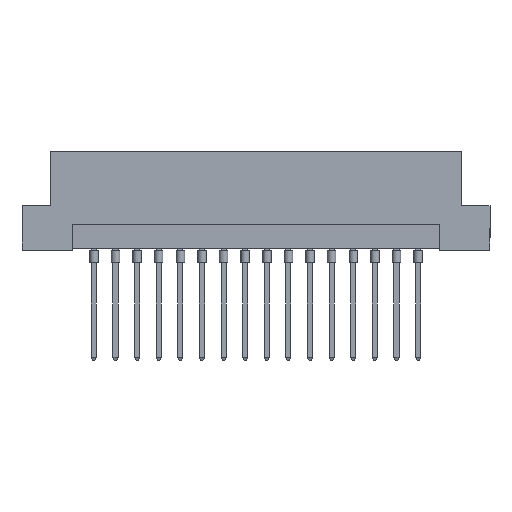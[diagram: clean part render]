
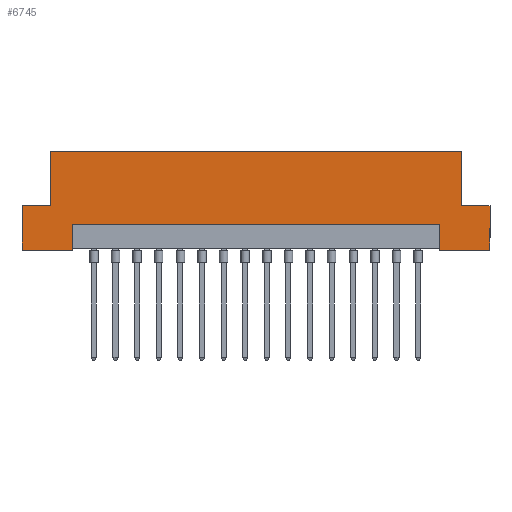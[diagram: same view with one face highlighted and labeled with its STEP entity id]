
A CAD part, front view. The second image highlights one B-rep face of the part: STEP entity #6745.
In plain terms, the highlighted planar face has unit normal (0, -1, 0).
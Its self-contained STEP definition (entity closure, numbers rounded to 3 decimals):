
#138 = VERTEX_POINT ( 'NONE', #5487 ) ;
#185 = CARTESIAN_POINT ( 'NONE',  ( -27.5, -4.3, 0. ) ) ;
#204 = VERTEX_POINT ( 'NONE', #851 ) ;
#213 = EDGE_CURVE ( 'NONE', #204, #7068, #4487, .T. ) ;
#248 = EDGE_CURVE ( 'NONE', #3055, #945, #3941, .T. ) ;
#302 = LINE ( 'NONE', #2579, #6960 ) ;
#372 = EDGE_CURVE ( 'NONE', #3192, #7068, #4767, .T. ) ;
#400 = DIRECTION ( 'NONE',  ( -1., 0., 0. ) ) ;
#407 = VECTOR ( 'NONE', #2073, 1000. ) ;
#435 = DIRECTION ( 'NONE',  ( 1., 0., 0. ) ) ;
#464 = EDGE_CURVE ( 'NONE', #3206, #4541, #3808, .T. ) ;
#480 = ORIENTED_EDGE ( 'NONE', *, *, #2262, .F. ) ;
#520 = CARTESIAN_POINT ( 'NONE',  ( -24.2, -4.3, 5.2 ) ) ;
#597 = ORIENTED_EDGE ( 'NONE', *, *, #213, .F. ) ;
#606 = DIRECTION ( 'NONE',  ( 1., 0., 0. ) ) ;
#626 = DIRECTION ( 'NONE',  ( 0., 0., -1. ) ) ;
#647 = ORIENTED_EDGE ( 'NONE', *, *, #3857, .F. ) ;
#851 = CARTESIAN_POINT ( 'NONE',  ( 21.6, -4.3, 0. ) ) ;
#887 = ORIENTED_EDGE ( 'NONE', *, *, #248, .T. ) ;
#945 = VERTEX_POINT ( 'NONE', #6007 ) ;
#1149 = CARTESIAN_POINT ( 'NONE',  ( -27.5, -4.3, 11.6 ) ) ;
#1151 = DIRECTION ( 'NONE',  ( 0., 0., 1. ) ) ;
#1225 = ORIENTED_EDGE ( 'NONE', *, *, #4520, .F. ) ;
#1260 = VECTOR ( 'NONE', #606, 1000. ) ;
#1372 = LINE ( 'NONE', #6908, #6774 ) ;
#1403 = EDGE_CURVE ( 'NONE', #3192, #945, #3871, .T. ) ;
#1470 = DIRECTION ( 'NONE',  ( 0., 0., 1. ) ) ;
#1485 = ORIENTED_EDGE ( 'NONE', *, *, #372, .T. ) ;
#1517 = DIRECTION ( 'NONE',  ( 1., 0., 0. ) ) ;
#1520 = ORIENTED_EDGE ( 'NONE', *, *, #1403, .F. ) ;
#1553 = CARTESIAN_POINT ( 'NONE',  ( 27.5, -4.3, 0. ) ) ;
#1644 = CARTESIAN_POINT ( 'NONE',  ( 24.2, -4.3, 5.2 ) ) ;
#1664 = ORIENTED_EDGE ( 'NONE', *, *, #6808, .T. ) ;
#1758 = EDGE_CURVE ( 'NONE', #4231, #3804, #3648, .T. ) ;
#1940 = FACE_OUTER_BOUND ( 'NONE', #5467, .T. ) ;
#1981 = VECTOR ( 'NONE', #5628, 1000. ) ;
#2043 = CARTESIAN_POINT ( 'NONE',  ( -21.6, -4.3, 3. ) ) ;
#2073 = DIRECTION ( 'NONE',  ( 1., 0., 0. ) ) ;
#2262 = EDGE_CURVE ( 'NONE', #4231, #3206, #302, .T. ) ;
#2272 = DIRECTION ( 'NONE',  ( 0., 0., -1. ) ) ;
#2413 = VERTEX_POINT ( 'NONE', #520 ) ;
#2546 = VECTOR ( 'NONE', #1470, 1000. ) ;
#2549 = DIRECTION ( 'NONE',  ( 1., 0., 0. ) ) ;
#2579 = CARTESIAN_POINT ( 'NONE',  ( 27.5, -4.3, 5.2 ) ) ;
#2624 = VECTOR ( 'NONE', #435, 1000. ) ;
#2743 = LINE ( 'NONE', #6588, #1981 ) ;
#2784 = VECTOR ( 'NONE', #1517, 1000. ) ;
#3055 = VERTEX_POINT ( 'NONE', #185 ) ;
#3159 = CARTESIAN_POINT ( 'NONE',  ( 24.2, -4.3, 5.2 ) ) ;
#3179 = CARTESIAN_POINT ( 'NONE',  ( -21.6, -4.3, 3. ) ) ;
#3192 = VERTEX_POINT ( 'NONE', #3179 ) ;
#3206 = VERTEX_POINT ( 'NONE', #7001 ) ;
#3353 = CARTESIAN_POINT ( 'NONE',  ( 27.5, -4.3, 0. ) ) ;
#3574 = DIRECTION ( 'NONE',  ( 0., 0., 1. ) ) ;
#3604 = DIRECTION ( 'NONE',  ( 0., 1., 0. ) ) ;
#3634 = LINE ( 'NONE', #7040, #407 ) ;
#3648 = LINE ( 'NONE', #3159, #2546 ) ;
#3804 = VERTEX_POINT ( 'NONE', #7167 ) ;
#3808 = LINE ( 'NONE', #6565, #7158 ) ;
#3857 = EDGE_CURVE ( 'NONE', #5501, #2413, #2743, .T. ) ;
#3871 = LINE ( 'NONE', #5454, #5777 ) ;
#3941 = LINE ( 'NONE', #3353, #1260 ) ;
#4032 = CARTESIAN_POINT ( 'NONE',  ( 21.6, -4.3, 3. ) ) ;
#4230 = AXIS2_PLACEMENT_3D ( 'NONE', #6348, #3604, #400 ) ;
#4231 = VERTEX_POINT ( 'NONE', #1644 ) ;
#4487 = LINE ( 'NONE', #6832, #7036 ) ;
#4520 = EDGE_CURVE ( 'NONE', #138, #3804, #7034, .T. ) ;
#4541 = VERTEX_POINT ( 'NONE', #1553 ) ;
#4767 = LINE ( 'NONE', #2043, #2624 ) ;
#5176 = DIRECTION ( 'NONE',  ( 0., 0., -1. ) ) ;
#5250 = CARTESIAN_POINT ( 'NONE',  ( -27.5, -4.3, 5.2 ) ) ;
#5270 = ORIENTED_EDGE ( 'NONE', *, *, #1758, .T. ) ;
#5454 = CARTESIAN_POINT ( 'NONE',  ( -21.6, -4.3, 0.2 ) ) ;
#5458 = ORIENTED_EDGE ( 'NONE', *, *, #5891, .F. ) ;
#5467 = EDGE_LOOP ( 'NONE', ( #1485, #597, #1664, #6492, #480, #5270, #1225, #5458, #647, #5688, #887, #1520 ) ) ;
#5487 = CARTESIAN_POINT ( 'NONE',  ( -24.2, -4.3, 11.6 ) ) ;
#5501 = VERTEX_POINT ( 'NONE', #5250 ) ;
#5603 = VECTOR ( 'NONE', #5176, 1000. ) ;
#5628 = DIRECTION ( 'NONE',  ( 1., 0., 0. ) ) ;
#5688 = ORIENTED_EDGE ( 'NONE', *, *, #5742, .T. ) ;
#5742 = EDGE_CURVE ( 'NONE', #5501, #3055, #6686, .T. ) ;
#5777 = VECTOR ( 'NONE', #2272, 1000. ) ;
#5837 = CARTESIAN_POINT ( 'NONE',  ( 27.5, -4.3, 11.6 ) ) ;
#5891 = EDGE_CURVE ( 'NONE', #2413, #138, #1372, .T. ) ;
#6007 = CARTESIAN_POINT ( 'NONE',  ( -21.6, -4.3, 0. ) ) ;
#6348 = CARTESIAN_POINT ( 'NONE',  ( 27.5, -4.3, 11.6 ) ) ;
#6492 = ORIENTED_EDGE ( 'NONE', *, *, #464, .F. ) ;
#6565 = CARTESIAN_POINT ( 'NONE',  ( 27.5, -4.3, 11.6 ) ) ;
#6588 = CARTESIAN_POINT ( 'NONE',  ( -27.5, -4.3, 5.2 ) ) ;
#6686 = LINE ( 'NONE', #1149, #5603 ) ;
#6745 = ADVANCED_FACE ( 'NONE', ( #1940 ), #6902, .F. ) ;
#6774 = VECTOR ( 'NONE', #3574, 1000. ) ;
#6808 = EDGE_CURVE ( 'NONE', #204, #4541, #3634, .T. ) ;
#6832 = CARTESIAN_POINT ( 'NONE',  ( 21.6, -4.3, 0.2 ) ) ;
#6902 = PLANE ( 'NONE',  #4230 ) ;
#6908 = CARTESIAN_POINT ( 'NONE',  ( -24.2, -4.3, 5.2 ) ) ;
#6960 = VECTOR ( 'NONE', #2549, 1000. ) ;
#7001 = CARTESIAN_POINT ( 'NONE',  ( 27.5, -4.3, 5.2 ) ) ;
#7034 = LINE ( 'NONE', #5837, #2784 ) ;
#7036 = VECTOR ( 'NONE', #1151, 1000. ) ;
#7040 = CARTESIAN_POINT ( 'NONE',  ( 27.5, -4.3, 0. ) ) ;
#7068 = VERTEX_POINT ( 'NONE', #4032 ) ;
#7158 = VECTOR ( 'NONE', #626, 1000. ) ;
#7167 = CARTESIAN_POINT ( 'NONE',  ( 24.2, -4.3, 11.6 ) ) ;
